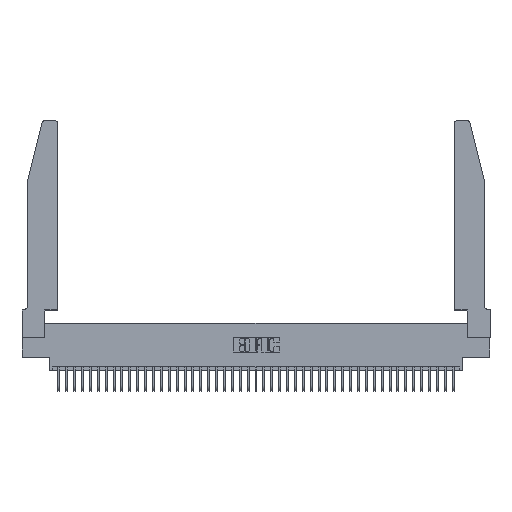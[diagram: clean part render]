
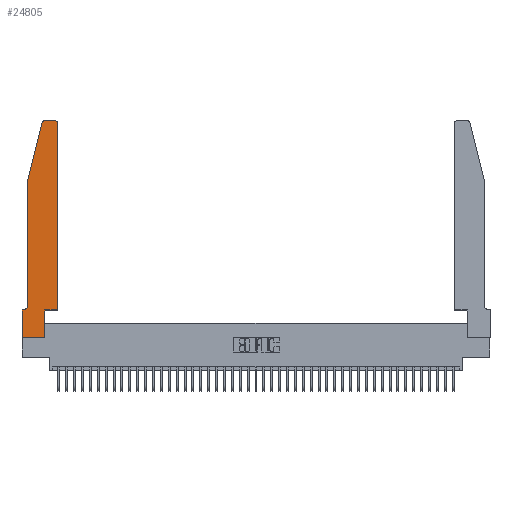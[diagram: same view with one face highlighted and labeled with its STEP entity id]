
A CAD part, top view. The second image highlights one B-rep face of the part: STEP entity #24805.
In plain terms, the highlighted planar face has unit normal (0, 0, 1).
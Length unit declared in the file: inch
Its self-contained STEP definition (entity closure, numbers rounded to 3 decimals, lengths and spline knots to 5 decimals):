
#273 = EDGE_CURVE ( 'NONE', #35687, #31951, #16249, .T. ) ;
#1014 = CARTESIAN_POINT ( 'NONE',  ( 0.2865, 0.35, 0.37 ) ) ;
#1713 = VERTEX_POINT ( 'NONE', #43721 ) ;
#1797 = AXIS2_PLACEMENT_3D ( 'NONE', #39606, #18767, #43103 ) ;
#2972 = ORIENTED_EDGE ( 'NONE', *, *, #29947, .T. ) ;
#3259 = FACE_OUTER_BOUND ( 'NONE', #25611, .T. ) ;
#3454 = CARTESIAN_POINT ( 'NONE',  ( 0., 0.35, 0.37 ) ) ;
#3911 = DIRECTION ( 'NONE',  ( 0., 1., 0. ) ) ;
#4243 = CARTESIAN_POINT ( 'NONE',  ( 0.4505, 0.35, 0.37 ) ) ;
#5252 = VECTOR ( 'NONE', #31201, 39.37008 ) ;
#6490 = EDGE_CURVE ( 'NONE', #14316, #21518, #41676, .T. ) ;
#6567 = VERTEX_POINT ( 'NONE', #7715 ) ;
#6767 = ORIENTED_EDGE ( 'NONE', *, *, #29410, .T. ) ;
#7097 = CARTESIAN_POINT ( 'NONE',  ( 0., 0., 0.37 ) ) ;
#7263 = CIRCLE ( 'NONE', #11597, 0.03 ) ;
#7402 = CARTESIAN_POINT ( 'NONE',  ( 0.284, 2.72, 0.37 ) ) ;
#7715 = CARTESIAN_POINT ( 'NONE',  ( 0.0755, 2., 0.37 ) ) ;
#7971 = LINE ( 'NONE', #7097, #25543 ) ;
#9163 = DIRECTION ( 'NONE',  ( -0.239, -0.971, 0. ) ) ;
#10621 = VERTEX_POINT ( 'NONE', #1014 ) ;
#10954 = DIRECTION ( 'NONE',  ( 1., 0., 0. ) ) ;
#11152 = ORIENTED_EDGE ( 'NONE', *, *, #273, .T. ) ;
#11597 = AXIS2_PLACEMENT_3D ( 'NONE', #36661, #15795, #40140 ) ;
#11910 = LINE ( 'NONE', #35877, #29403 ) ;
#12139 = DIRECTION ( 'NONE',  ( -1., 0., 0. ) ) ;
#12418 = CARTESIAN_POINT ( 'NONE',  ( 0.284, 2.75, 0.37 ) ) ;
#13380 = DIRECTION ( 'NONE',  ( 1., 0., 0. ) ) ;
#13615 = CARTESIAN_POINT ( 'NONE',  ( 0.2605, 2.75, 0.37 ) ) ;
#13680 = ORIENTED_EDGE ( 'NONE', *, *, #40980, .T. ) ;
#13947 = ORIENTED_EDGE ( 'NONE', *, *, #23681, .T. ) ;
#14316 = VERTEX_POINT ( 'NONE', #12418 ) ;
#14686 = LINE ( 'NONE', #26643, #22898 ) ;
#15249 = PLANE ( 'NONE',  #1797 ) ;
#15795 = DIRECTION ( 'NONE',  ( 0., 0., 1. ) ) ;
#16249 = LINE ( 'NONE', #33025, #26634 ) ;
#16418 = VECTOR ( 'NONE', #3911, 39.37008 ) ;
#17497 = EDGE_CURVE ( 'NONE', #19780, #35687, #43212, .T. ) ;
#18767 = DIRECTION ( 'NONE',  ( 0., 0., 1. ) ) ;
#19780 = VERTEX_POINT ( 'NONE', #34321 ) ;
#20729 = ORIENTED_EDGE ( 'NONE', *, *, #6490, .T. ) ;
#20953 = CARTESIAN_POINT ( 'NONE',  ( 0.0055, 0.42, 0.37 ) ) ;
#21271 = EDGE_CURVE ( 'NONE', #1713, #42658, #43534, .T. ) ;
#21518 = VERTEX_POINT ( 'NONE', #39533 ) ;
#22267 = CARTESIAN_POINT ( 'NONE',  ( 0.4205, 2.75, 0.37 ) ) ;
#22898 = VECTOR ( 'NONE', #9163, 39.37008 ) ;
#23681 = EDGE_CURVE ( 'NONE', #26218, #37884, #7263, .T. ) ;
#24494 = DIRECTION ( 'NONE',  ( -1., 0., 0. ) ) ;
#24805 = ADVANCED_FACE ( 'NONE', ( #3259 ), #15249, .T. ) ;
#24953 = ORIENTED_EDGE ( 'NONE', *, *, #27973, .T. ) ;
#25543 = VECTOR ( 'NONE', #28090, 39.37008 ) ;
#25611 = EDGE_LOOP ( 'NONE', ( #13680, #20729, #37194, #24953, #39963, #11152, #6767, #36199, #40994, #2972, #37249, #13947 ) ) ;
#25710 = LINE ( 'NONE', #28483, #16418 ) ;
#26005 = CARTESIAN_POINT ( 'NONE',  ( 0.4505, 2.72, 0.37 ) ) ;
#26218 = VERTEX_POINT ( 'NONE', #26005 ) ;
#26634 = VECTOR ( 'NONE', #12139, 39.37008 ) ;
#26643 = CARTESIAN_POINT ( 'NONE',  ( 0.0755, 2., 0.37 ) ) ;
#27723 = AXIS2_PLACEMENT_3D ( 'NONE', #7402, #31868, #10954 ) ;
#27973 = EDGE_CURVE ( 'NONE', #6567, #19780, #11910, .T. ) ;
#27983 = LINE ( 'NONE', #31662, #45366 ) ;
#28090 = DIRECTION ( 'NONE',  ( 0., -1., 0. ) ) ;
#28483 = CARTESIAN_POINT ( 'NONE',  ( 0.4505, 0.35, 0.37 ) ) ;
#29403 = VECTOR ( 'NONE', #39383, 39.37008 ) ;
#29410 = EDGE_CURVE ( 'NONE', #31951, #1713, #7971, .T. ) ;
#29947 = EDGE_CURVE ( 'NONE', #10621, #43122, #43964, .T. ) ;
#30782 = CARTESIAN_POINT ( 'NONE',  ( 0.4505, 0.35, 0.37 ) ) ;
#31201 = DIRECTION ( 'NONE',  ( 1., 0., 0. ) ) ;
#31662 = CARTESIAN_POINT ( 'NONE',  ( 0.2865, 0.35, 0.37 ) ) ;
#31868 = DIRECTION ( 'NONE',  ( 0., 0., 1. ) ) ;
#31951 = VERTEX_POINT ( 'NONE', #3454 ) ;
#31993 = EDGE_CURVE ( 'NONE', #42658, #10621, #27983, .T. ) ;
#32449 = CARTESIAN_POINT ( 'NONE',  ( 0.2865, 0., 0.37 ) ) ;
#33025 = CARTESIAN_POINT ( 'NONE',  ( 0.0755, 0.35, 0.37 ) ) ;
#34321 = CARTESIAN_POINT ( 'NONE',  ( 0.0755, 0.42, 0.37 ) ) ;
#34701 = CARTESIAN_POINT ( 'NONE',  ( 0., 0., 0.37 ) ) ;
#35223 = VECTOR ( 'NONE', #44987, 39.37008 ) ;
#35687 = VERTEX_POINT ( 'NONE', #45098 ) ;
#35877 = CARTESIAN_POINT ( 'NONE',  ( 0.0755, 2., 0.37 ) ) ;
#36199 = ORIENTED_EDGE ( 'NONE', *, *, #21271, .T. ) ;
#36661 = CARTESIAN_POINT ( 'NONE',  ( 0.4205, 2.72, 0.37 ) ) ;
#37194 = ORIENTED_EDGE ( 'NONE', *, *, #38737, .T. ) ;
#37249 = ORIENTED_EDGE ( 'NONE', *, *, #44864, .T. ) ;
#37884 = VERTEX_POINT ( 'NONE', #22267 ) ;
#38664 = DIRECTION ( 'NONE',  ( 0., 1., 0. ) ) ;
#38737 = EDGE_CURVE ( 'NONE', #21518, #6567, #14686, .T. ) ;
#39383 = DIRECTION ( 'NONE',  ( 0., -1., 0. ) ) ;
#39533 = CARTESIAN_POINT ( 'NONE',  ( 0.25487, 2.72718, 0.37 ) ) ;
#39606 = CARTESIAN_POINT ( 'NONE',  ( 0., 0.35, 0.37 ) ) ;
#39963 = ORIENTED_EDGE ( 'NONE', *, *, #17497, .T. ) ;
#40140 = DIRECTION ( 'NONE',  ( 1., 0., 0. ) ) ;
#40980 = EDGE_CURVE ( 'NONE', #37884, #14316, #44454, .T. ) ;
#40994 = ORIENTED_EDGE ( 'NONE', *, *, #31993, .T. ) ;
#41676 = CIRCLE ( 'NONE', #27723, 0.03 ) ;
#42358 = AXIS2_PLACEMENT_3D ( 'NONE', #20953, #45293, #24494 ) ;
#42658 = VERTEX_POINT ( 'NONE', #32449 ) ;
#42873 = VECTOR ( 'NONE', #13380, 39.37008 ) ;
#43103 = DIRECTION ( 'NONE',  ( 1., 0., 0. ) ) ;
#43122 = VERTEX_POINT ( 'NONE', #4243 ) ;
#43212 = CIRCLE ( 'NONE', #42358, 0.07 ) ;
#43534 = LINE ( 'NONE', #34701, #5252 ) ;
#43721 = CARTESIAN_POINT ( 'NONE',  ( 0., 0., 0.37 ) ) ;
#43964 = LINE ( 'NONE', #30782, #42873 ) ;
#44454 = LINE ( 'NONE', #13615, #35223 ) ;
#44864 = EDGE_CURVE ( 'NONE', #43122, #26218, #25710, .T. ) ;
#44987 = DIRECTION ( 'NONE',  ( -1., 0., 0. ) ) ;
#45098 = CARTESIAN_POINT ( 'NONE',  ( 0.0055, 0.35, 0.37 ) ) ;
#45293 = DIRECTION ( 'NONE',  ( 0., 0., -1. ) ) ;
#45366 = VECTOR ( 'NONE', #38664, 39.37008 ) ;
